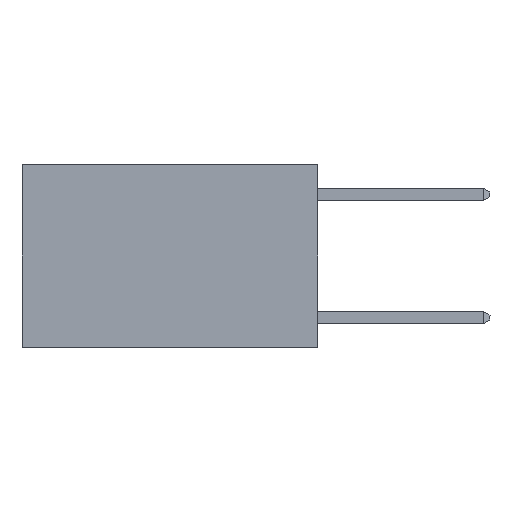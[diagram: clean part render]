
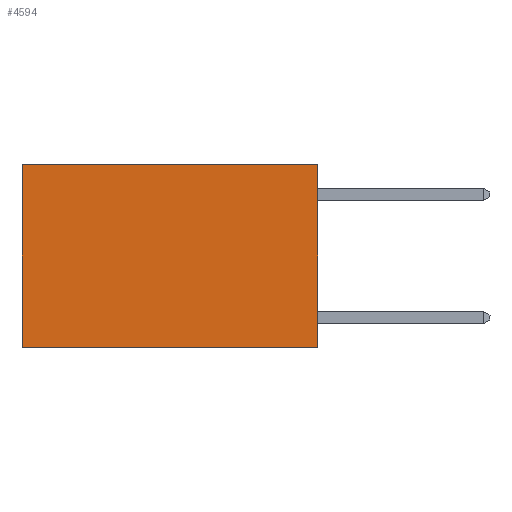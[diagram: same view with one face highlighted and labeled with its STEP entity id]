
A CAD part, left-side view. The second image highlights one B-rep face of the part: STEP entity #4594.
In plain terms, the highlighted planar face has unit normal (-1, 0, 0).
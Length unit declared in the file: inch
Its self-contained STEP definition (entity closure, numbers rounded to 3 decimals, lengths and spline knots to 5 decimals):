
#120 = CARTESIAN_POINT ( 'NONE',  ( 0.2625, 0.6, -0.37 ) ) ;
#234 = VERTEX_POINT ( 'NONE', #6132 ) ;
#846 = VERTEX_POINT ( 'NONE', #3197 ) ;
#1043 = EDGE_LOOP ( 'NONE', ( #7241, #7356, #2478, #1795 ) ) ;
#1795 = ORIENTED_EDGE ( 'NONE', *, *, #3459, .T. ) ;
#1851 = LINE ( 'NONE', #8870, #3654 ) ;
#2349 = VECTOR ( 'NONE', #9206, 39.37008 ) ;
#2478 = ORIENTED_EDGE ( 'NONE', *, *, #3506, .F. ) ;
#2701 = DIRECTION ( 'NONE',  ( 0., 0., -1. ) ) ;
#2709 = DIRECTION ( 'NONE',  ( 1., 0., 0. ) ) ;
#2741 = PLANE ( 'NONE',  #6536 ) ;
#2896 = CARTESIAN_POINT ( 'NONE',  ( 0.2625, 0., 0. ) ) ;
#3079 = VECTOR ( 'NONE', #9323, 39.37008 ) ;
#3197 = CARTESIAN_POINT ( 'NONE',  ( 0.2625, 0., 0. ) ) ;
#3459 = EDGE_CURVE ( 'NONE', #846, #6286, #4593, .T. ) ;
#3506 = EDGE_CURVE ( 'NONE', #846, #234, #6454, .T. ) ;
#3616 = EDGE_CURVE ( 'NONE', #6286, #5900, #1851, .T. ) ;
#3654 = VECTOR ( 'NONE', #8757, 39.37008 ) ;
#4311 = LINE ( 'NONE', #7783, #7792 ) ;
#4593 = LINE ( 'NONE', #9353, #3079 ) ;
#4594 = ADVANCED_FACE ( 'NONE', ( #8115 ), #2741, .F. ) ;
#5403 = EDGE_CURVE ( 'NONE', #234, #5900, #4311, .T. ) ;
#5900 = VERTEX_POINT ( 'NONE', #120 ) ;
#6132 = CARTESIAN_POINT ( 'NONE',  ( 0.2625, 0., -0.37 ) ) ;
#6286 = VERTEX_POINT ( 'NONE', #8764 ) ;
#6454 = LINE ( 'NONE', #9152, #2349 ) ;
#6536 = AXIS2_PLACEMENT_3D ( 'NONE', #2896, #2709, #2701 ) ;
#7241 = ORIENTED_EDGE ( 'NONE', *, *, #3616, .T. ) ;
#7356 = ORIENTED_EDGE ( 'NONE', *, *, #5403, .F. ) ;
#7696 = DIRECTION ( 'NONE',  ( 0., 1., 0. ) ) ;
#7783 = CARTESIAN_POINT ( 'NONE',  ( 0.2625, 0., -0.37 ) ) ;
#7792 = VECTOR ( 'NONE', #7696, 39.37008 ) ;
#8115 = FACE_OUTER_BOUND ( 'NONE', #1043, .T. ) ;
#8757 = DIRECTION ( 'NONE',  ( 0., 0., -1. ) ) ;
#8764 = CARTESIAN_POINT ( 'NONE',  ( 0.2625, 0.6, 0. ) ) ;
#8870 = CARTESIAN_POINT ( 'NONE',  ( 0.2625, 0.6, 0. ) ) ;
#9152 = CARTESIAN_POINT ( 'NONE',  ( 0.2625, 0., 0. ) ) ;
#9206 = DIRECTION ( 'NONE',  ( 0., 0., -1. ) ) ;
#9323 = DIRECTION ( 'NONE',  ( 0., 1., 0. ) ) ;
#9353 = CARTESIAN_POINT ( 'NONE',  ( 0.2625, 0., 0. ) ) ;
